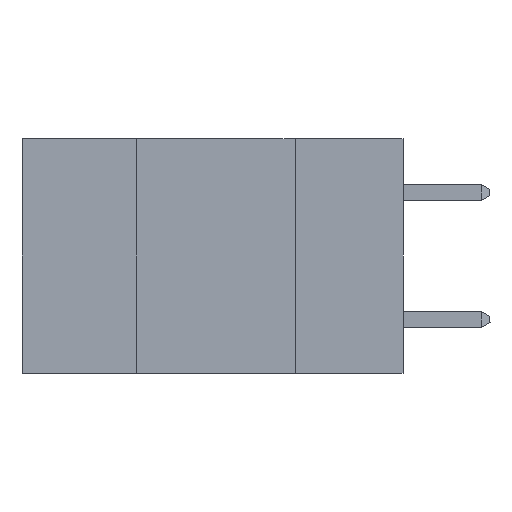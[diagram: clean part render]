
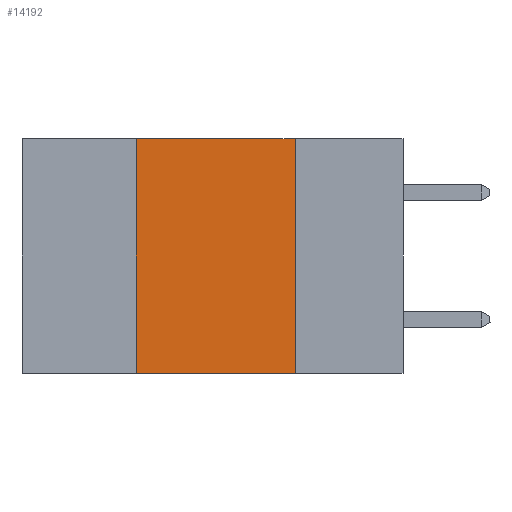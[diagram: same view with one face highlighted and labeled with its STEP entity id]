
A CAD part, left-side view. The second image highlights one B-rep face of the part: STEP entity #14192.
In plain terms, the highlighted planar face has unit normal (-1, 0, 0).
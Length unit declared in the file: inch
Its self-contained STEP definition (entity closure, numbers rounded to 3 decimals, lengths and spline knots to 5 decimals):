
#301 = PLANE ( 'NONE',  #9152 ) ;
#1444 = EDGE_LOOP ( 'NONE', ( #7021, #11954, #16528, #18613 ) ) ;
#2250 = VECTOR ( 'NONE', #12604, 39.37008 ) ;
#2469 = CARTESIAN_POINT ( 'NONE',  ( 0., 0.6, 0. ) ) ;
#2715 = LINE ( 'NONE', #2469, #2250 ) ;
#2780 = FACE_OUTER_BOUND ( 'NONE', #1444, .T. ) ;
#3247 = DIRECTION ( 'NONE',  ( 1., 0., 0. ) ) ;
#3301 = VERTEX_POINT ( 'NONE', #10579 ) ;
#3585 = EDGE_CURVE ( 'NONE', #11256, #3301, #14795, .T. ) ;
#3676 = DIRECTION ( 'NONE',  ( 0., -1., 0. ) ) ;
#3775 = CARTESIAN_POINT ( 'NONE',  ( 0., 0.42, 0. ) ) ;
#4478 = CARTESIAN_POINT ( 'NONE',  ( 0., 0.17, 0. ) ) ;
#5033 = EDGE_CURVE ( 'NONE', #16478, #7911, #2715, .T. ) ;
#6157 = CARTESIAN_POINT ( 'NONE',  ( 0., 0.6, -0.37 ) ) ;
#6687 = EDGE_CURVE ( 'NONE', #7911, #3301, #10785, .T. ) ;
#7021 = ORIENTED_EDGE ( 'NONE', *, *, #6687, .F. ) ;
#7153 = VECTOR ( 'NONE', #3676, 39.37008 ) ;
#7756 = DIRECTION ( 'NONE',  ( 0., 0., -1. ) ) ;
#7911 = VERTEX_POINT ( 'NONE', #4478 ) ;
#9152 = AXIS2_PLACEMENT_3D ( 'NONE', #16265, #3247, #13393 ) ;
#9274 = DIRECTION ( 'NONE',  ( 0., 0., 1. ) ) ;
#9540 = CARTESIAN_POINT ( 'NONE',  ( 0., 0.42, -0.37 ) ) ;
#10579 = CARTESIAN_POINT ( 'NONE',  ( 0., 0.17, -0.37 ) ) ;
#10785 = LINE ( 'NONE', #17865, #11242 ) ;
#11242 = VECTOR ( 'NONE', #7756, 39.37008 ) ;
#11256 = VERTEX_POINT ( 'NONE', #9540 ) ;
#11954 = ORIENTED_EDGE ( 'NONE', *, *, #5033, .F. ) ;
#12103 = VECTOR ( 'NONE', #9274, 39.37008 ) ;
#12559 = LINE ( 'NONE', #13574, #12103 ) ;
#12604 = DIRECTION ( 'NONE',  ( 0., -1., 0. ) ) ;
#13393 = DIRECTION ( 'NONE',  ( 0., 0., -1. ) ) ;
#13574 = CARTESIAN_POINT ( 'NONE',  ( 0., 0.42, 0. ) ) ;
#14192 = ADVANCED_FACE ( 'NONE', ( #2780 ), #301, .F. ) ;
#14795 = LINE ( 'NONE', #6157, #7153 ) ;
#16265 = CARTESIAN_POINT ( 'NONE',  ( 0., 0.6, 0. ) ) ;
#16478 = VERTEX_POINT ( 'NONE', #3775 ) ;
#16528 = ORIENTED_EDGE ( 'NONE', *, *, #18773, .F. ) ;
#17865 = CARTESIAN_POINT ( 'NONE',  ( 0., 0.17, 0. ) ) ;
#18613 = ORIENTED_EDGE ( 'NONE', *, *, #3585, .T. ) ;
#18773 = EDGE_CURVE ( 'NONE', #11256, #16478, #12559, .T. ) ;
